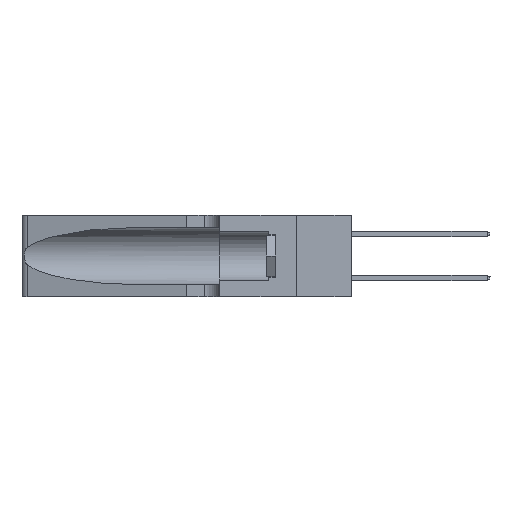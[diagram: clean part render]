
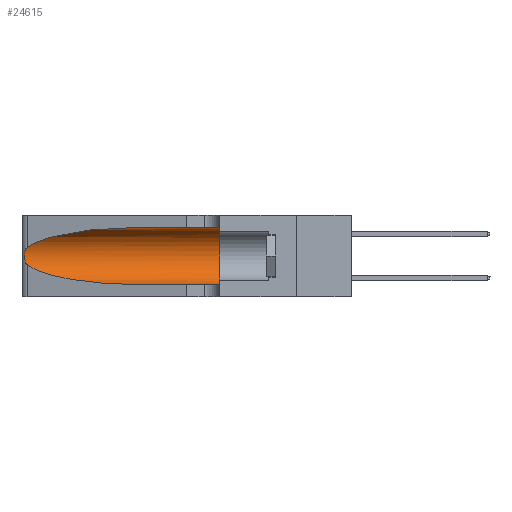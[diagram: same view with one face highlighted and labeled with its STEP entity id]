
A CAD part, left-side view. The second image highlights one B-rep face of the part: STEP entity #24615.
In plain terms, the highlighted cylindrical face has radius 3.308 mm (diameter 6.617 mm), a partial arc.
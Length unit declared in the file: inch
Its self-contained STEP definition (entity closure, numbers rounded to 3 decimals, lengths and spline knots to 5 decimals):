
#152 = CARTESIAN_POINT ( 'NONE',  ( 0.25639, 1.23186, 0.15144 ) ) ;
#189 = DIRECTION ( 'NONE',  ( 0., -1., 0. ) ) ;
#496 = CARTESIAN_POINT ( 'NONE',  ( 0.1305, 1.61858, 0.05475 ) ) ;
#589 = DIRECTION ( 'NONE',  ( 0., -1., 0. ) ) ;
#1061 = LINE ( 'NONE', #496, #25840 ) ;
#1164 = VERTEX_POINT ( 'NONE', #17564 ) ;
#1582 = CYLINDRICAL_SURFACE ( 'NONE', #7902, 0.13025 ) ;
#2419 = CARTESIAN_POINT ( 'NONE',  ( 0.25487, 1.22718, 0.22369 ) ) ;
#2429 = CARTESIAN_POINT ( 'NONE',  ( 0.1305, 1.61858, 0.185 ) ) ;
#2626 = CARTESIAN_POINT ( 'NONE',  ( 0.25787, 1.23484, 0.2124 ) ) ;
#2949 = DIRECTION ( 'NONE',  ( 0., 0., -1. ) ) ;
#3014 = ORIENTED_EDGE ( 'NONE', *, *, #26550, .T. ) ;
#3501 = ORIENTED_EDGE ( 'NONE', *, *, #7156, .T. ) ;
#3699 = VERTEX_POINT ( 'NONE', #10736 ) ;
#3974 = CARTESIAN_POINT ( 'NONE',  ( 0.1305, 0.35, 0.185 ) ) ;
#4904 = CARTESIAN_POINT ( 'NONE',  ( 0.26017, 1.23833, 0.17102 ) ) ;
#5111 = CARTESIAN_POINT ( 'NONE',  ( 0.26075, 1.23896, 0.178 ) ) ;
#5343 = CARTESIAN_POINT ( 'NONE',  ( 0.18966, 0.96281, 0.31525 ) ) ;
#5378 = ORIENTED_EDGE ( 'NONE', *, *, #5638, .F. ) ;
#5410 = CARTESIAN_POINT ( 'NONE',  ( 0.1305, 0.35, 0.31525 ) ) ;
#5638 = EDGE_CURVE ( 'NONE', #1164, #8285, #16477, .T. ) ;
#6346 = CARTESIAN_POINT ( 'NONE',  ( 0.1305, 1.61858, 0.31525 ) ) ;
#7156 = EDGE_CURVE ( 'NONE', #13707, #19594, #28444, .T. ) ;
#7392 = ORIENTED_EDGE ( 'NONE', *, *, #26143, .T. ) ;
#7521 = CARTESIAN_POINT ( 'NONE',  ( 0.25639, 1.23184, 0.21858 ) ) ;
#7902 = AXIS2_PLACEMENT_3D ( 'NONE', #2429, #589, #2949 ) ;
#8285 = VERTEX_POINT ( 'NONE', #5410 ) ;
#9185 = CIRCLE ( 'NONE', #29533, 0.13025 ) ;
#9677 = CARTESIAN_POINT ( 'NONE',  ( 0.26018, 1.23835, 0.19895 ) ) ;
#9701 = CARTESIAN_POINT ( 'NONE',  ( 0.2373, 1.15595, 0.28018 ) ) ;
#10587 = EDGE_LOOP ( 'NONE', ( #3014, #3501, #7392, #11680, #19325, #5378 ) ) ;
#10736 = CARTESIAN_POINT ( 'NONE',  ( 0.1305, 0.72297, 0.05475 ) ) ;
#10812 = DIRECTION ( 'NONE',  ( 0., 1., 0. ) ) ;
#11680 = ORIENTED_EDGE ( 'NONE', *, *, #19578, .T. ) ;
#11969 = CARTESIAN_POINT ( 'NONE',  ( 0.25555, 1.22993, 0.14849 ) ) ;
#12076 = CARTESIAN_POINT ( 'NONE',  ( 0.25487, 1.22718, 0.14631 ) ) ;
#12308 = CARTESIAN_POINT ( 'NONE',  ( 0.25487, 1.22718, 0.22369 ) ) ;
#13051 = CARTESIAN_POINT ( 'NONE',  ( 0.25487, 1.22718, 0.22369 ) ) ;
#13707 = VERTEX_POINT ( 'NONE', #13051 ) ;
#14347 = CARTESIAN_POINT ( 'NONE',  ( 0.26075, 1.23896, 0.19203 ) ) ;
#15296 = FACE_OUTER_BOUND ( 'NONE', #10587, .T. ) ;
#15335 = CARTESIAN_POINT ( 'NONE',  ( 0.1305, 0.72297, 0.05475 ) ) ;
#15669 = DIRECTION ( 'NONE',  ( 0., -1., 0. ) ) ;
#16477 = LINE ( 'NONE', #6346, #17209 ) ;
#16988 = CARTESIAN_POINT ( 'NONE',  ( 0.1305, 0.35, 0.05475 ) ) ;
#17209 = VECTOR ( 'NONE', #15669, 39.37008 ) ;
#17564 = CARTESIAN_POINT ( 'NONE',  ( 0.1305, 0.72297, 0.31525 ) ) ;
#19027 = CARTESIAN_POINT ( 'NONE',  ( 0.25789, 1.23486, 0.15765 ) ) ;
#19127 = CARTESIAN_POINT ( 'NONE',  ( 0.25854, 1.2359, 0.20912 ) ) ;
#19325 = ORIENTED_EDGE ( 'NONE', *, *, #19725, .F. ) ;
#19430 = CARTESIAN_POINT ( 'NONE',  ( 0.25555, 1.22994, 0.2215 ) ) ;
#19578 = EDGE_CURVE ( 'NONE', #3699, #21107, #1061, .T. ) ;
#19594 = VERTEX_POINT ( 'NONE', #22064 ) ;
#19725 = EDGE_CURVE ( 'NONE', #8285, #21107, #9185, .T. ) ;
#19769 =( BOUNDED_CURVE ( )  B_SPLINE_CURVE ( 3, ( #27384, #24916, #20213, #15335 ),
 .UNSPECIFIED., .F., .F. ) 
 B_SPLINE_CURVE_WITH_KNOTS ( ( 4, 4 ),
 ( 3.44316, 4.71239 ),
 .UNSPECIFIED. ) 
 CURVE ( )  GEOMETRIC_REPRESENTATION_ITEM ( )  RATIONAL_B_SPLINE_CURVE ( ( 1., 0.87, 0.87, 1. ) ) 
 REPRESENTATION_ITEM ( '' )  );
#20213 = CARTESIAN_POINT ( 'NONE',  ( 0.18966, 0.96281, 0.05475 ) ) ;
#20772 = DIRECTION ( 'NONE',  ( 0., 0., 1. ) ) ;
#21107 = VERTEX_POINT ( 'NONE', #16988 ) ;
#22064 = CARTESIAN_POINT ( 'NONE',  ( 0.25487, 1.22718, 0.14631 ) ) ;
#24615 = ADVANCED_FACE ( 'NONE', ( #15296 ), #1582, .F. ) ;
#24916 = CARTESIAN_POINT ( 'NONE',  ( 0.2373, 1.15595, 0.08982 ) ) ;
#25611 =( BOUNDED_CURVE ( )  B_SPLINE_CURVE ( 3, ( #28739, #5343, #9701, #12308 ),
 .UNSPECIFIED., .F., .T. ) 
 B_SPLINE_CURVE_WITH_KNOTS ( ( 4, 4 ),
 ( 1.5708, 2.84003 ),
 .UNSPECIFIED. ) 
 CURVE ( )  GEOMETRIC_REPRESENTATION_ITEM ( )  RATIONAL_B_SPLINE_CURVE ( ( 1., 0.87, 0.87, 1. ) ) 
 REPRESENTATION_ITEM ( '' )  );
#25840 = VECTOR ( 'NONE', #189, 39.37008 ) ;
#26143 = EDGE_CURVE ( 'NONE', #19594, #3699, #19769, .T. ) ;
#26550 = EDGE_CURVE ( 'NONE', #1164, #13707, #25611, .T. ) ;
#27384 = CARTESIAN_POINT ( 'NONE',  ( 0.25487, 1.22718, 0.14631 ) ) ;
#28444 = B_SPLINE_CURVE_WITH_KNOTS ( 'NONE', 3,
 ( #2419, #19430, #7521, #2626, #19127, #9677, #14347, #5111, #4904, #28811, #19027, #152, #11969, #12076 ),
 .UNSPECIFIED., .F., .F.,
 ( 4, 2, 2, 2, 2, 2, 4 ),
 ( 0., 0.00027, 0.00053, 0.00107, 0.0016, 0.00187, 0.00214 ),
 .UNSPECIFIED. ) ;
#28739 = CARTESIAN_POINT ( 'NONE',  ( 0.1305, 0.72297, 0.31525 ) ) ;
#28811 = CARTESIAN_POINT ( 'NONE',  ( 0.25856, 1.23593, 0.16098 ) ) ;
#29533 = AXIS2_PLACEMENT_3D ( 'NONE', #3974, #10812, #20772 ) ;
